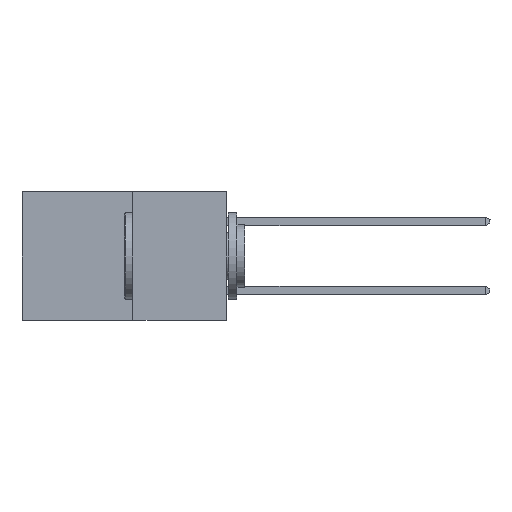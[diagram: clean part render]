
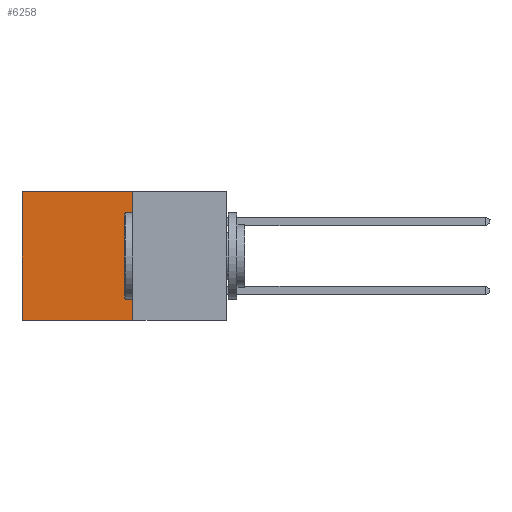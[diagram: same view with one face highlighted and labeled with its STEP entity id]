
A CAD part, left-side view. The second image highlights one B-rep face of the part: STEP entity #6258.
In plain terms, the highlighted planar face has unit normal (-1, 0, 0).
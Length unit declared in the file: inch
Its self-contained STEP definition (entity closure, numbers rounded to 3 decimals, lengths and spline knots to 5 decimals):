
#248 = DIRECTION ( 'NONE',  ( 0., 0., -1. ) ) ;
#274 = DIRECTION ( 'NONE',  ( 1., 0., 0. ) ) ;
#294 = CARTESIAN_POINT ( 'NONE',  ( 0.277, 0.27, -0.37 ) ) ;
#519 = PLANE ( 'NONE',  #20039 ) ;
#739 = ORIENTED_EDGE ( 'NONE', *, *, #8132, .F. ) ;
#2025 = CARTESIAN_POINT ( 'NONE',  ( 0.277, 0.27, 0. ) ) ;
#4056 = ORIENTED_EDGE ( 'NONE', *, *, #7099, .F. ) ;
#4134 = VECTOR ( 'NONE', #6324, 39.37008 ) ;
#4704 = EDGE_LOOP ( 'NONE', ( #19992, #4056, #739, #7468 ) ) ;
#6258 = ADVANCED_FACE ( 'NONE', ( #7068 ), #519, .F. ) ;
#6324 = DIRECTION ( 'NONE',  ( 0., 1., 0. ) ) ;
#7003 = EDGE_CURVE ( 'NONE', #24833, #14572, #23086, .T. ) ;
#7068 = FACE_OUTER_BOUND ( 'NONE', #4704, .T. ) ;
#7099 = EDGE_CURVE ( 'NONE', #17271, #14572, #15799, .T. ) ;
#7162 = VECTOR ( 'NONE', #8269, 39.37008 ) ;
#7468 = ORIENTED_EDGE ( 'NONE', *, *, #24149, .T. ) ;
#8119 = VECTOR ( 'NONE', #14051, 39.37008 ) ;
#8132 = EDGE_CURVE ( 'NONE', #10290, #17271, #8783, .T. ) ;
#8269 = DIRECTION ( 'NONE',  ( 0., 0., -1. ) ) ;
#8287 = CARTESIAN_POINT ( 'NONE',  ( 0.277, 0.59, -0.37 ) ) ;
#8617 = CARTESIAN_POINT ( 'NONE',  ( 0.277, 0.59, 0. ) ) ;
#8783 = LINE ( 'NONE', #14720, #8119 ) ;
#9466 = CARTESIAN_POINT ( 'NONE',  ( 0.277, 0.27, -0.37 ) ) ;
#10182 = VECTOR ( 'NONE', #10439, 39.37008 ) ;
#10290 = VERTEX_POINT ( 'NONE', #14631 ) ;
#10439 = DIRECTION ( 'NONE',  ( 0., 1., 0. ) ) ;
#10476 = LINE ( 'NONE', #2025, #4134 ) ;
#14051 = DIRECTION ( 'NONE',  ( 0., 0., -1. ) ) ;
#14572 = VERTEX_POINT ( 'NONE', #18514 ) ;
#14631 = CARTESIAN_POINT ( 'NONE',  ( 0.277, 0.27, 0. ) ) ;
#14720 = CARTESIAN_POINT ( 'NONE',  ( 0.277, 0.27, -0.37 ) ) ;
#15799 = LINE ( 'NONE', #9466, #10182 ) ;
#17271 = VERTEX_POINT ( 'NONE', #17591 ) ;
#17591 = CARTESIAN_POINT ( 'NONE',  ( 0.277, 0.27, -0.37 ) ) ;
#18514 = CARTESIAN_POINT ( 'NONE',  ( 0.277, 0.59, -0.37 ) ) ;
#19992 = ORIENTED_EDGE ( 'NONE', *, *, #7003, .T. ) ;
#20039 = AXIS2_PLACEMENT_3D ( 'NONE', #294, #274, #248 ) ;
#23086 = LINE ( 'NONE', #8287, #7162 ) ;
#24149 = EDGE_CURVE ( 'NONE', #10290, #24833, #10476, .T. ) ;
#24833 = VERTEX_POINT ( 'NONE', #8617 ) ;
